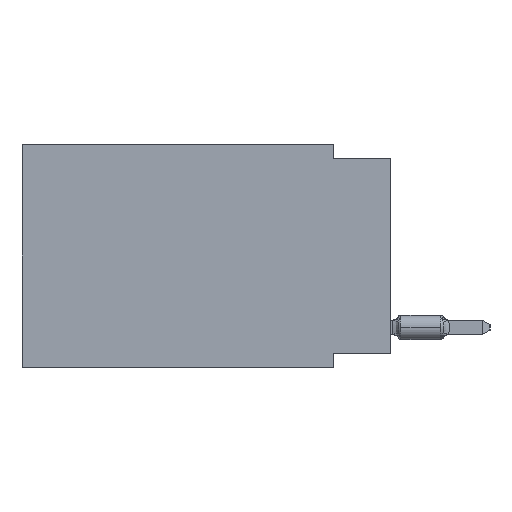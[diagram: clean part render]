
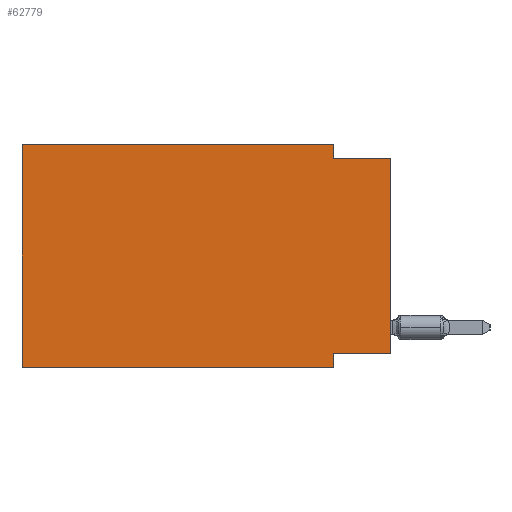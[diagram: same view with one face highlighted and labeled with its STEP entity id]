
A CAD part, left-side view. The second image highlights one B-rep face of the part: STEP entity #62779.
In plain terms, the highlighted planar face has unit normal (-1, 0, 0).
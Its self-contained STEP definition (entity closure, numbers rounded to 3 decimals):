
#2422 = LINE ( 'NONE', #65793, #82932 ) ;
#3543 = VERTEX_POINT ( 'NONE', #17332 ) ;
#3724 = VECTOR ( 'NONE', #83323, 1000. ) ;
#5546 = VECTOR ( 'NONE', #24853, 1000. ) ;
#5785 = CARTESIAN_POINT ( 'NONE',  ( 0., 2.54, -9.906 ) ) ;
#6326 = DIRECTION ( 'NONE',  ( 0., 1., 0. ) ) ;
#7982 = ORIENTED_EDGE ( 'NONE', *, *, #25823, .F. ) ;
#8582 = CARTESIAN_POINT ( 'NONE',  ( 0., 16.383, 0. ) ) ;
#11680 = CARTESIAN_POINT ( 'NONE',  ( 0., 16.383, -9.906 ) ) ;
#12291 = EDGE_CURVE ( 'NONE', #80662, #3543, #40938, .T. ) ;
#12907 = CARTESIAN_POINT ( 'NONE',  ( 0., 0., -9.271 ) ) ;
#14460 = CARTESIAN_POINT ( 'NONE',  ( 0., 2.54, 0. ) ) ;
#17332 = CARTESIAN_POINT ( 'NONE',  ( 0., 0., -0.635 ) ) ;
#18930 = AXIS2_PLACEMENT_3D ( 'NONE', #26075, #39243, #77903 ) ;
#21151 = ORIENTED_EDGE ( 'NONE', *, *, #24171, .T. ) ;
#23158 = CARTESIAN_POINT ( 'NONE',  ( 0., 2.54, -9.271 ) ) ;
#24171 = EDGE_CURVE ( 'NONE', #58174, #3543, #51066, .T. ) ;
#24853 = DIRECTION ( 'NONE',  ( 0., -1., 0. ) ) ;
#25823 = EDGE_CURVE ( 'NONE', #58174, #58140, #58614, .T. ) ;
#26075 = CARTESIAN_POINT ( 'NONE',  ( 0., 16.383, 0. ) ) ;
#26923 = CARTESIAN_POINT ( 'NONE',  ( 0., 0., -0.635 ) ) ;
#29465 = ORIENTED_EDGE ( 'NONE', *, *, #46650, .F. ) ;
#30961 = VERTEX_POINT ( 'NONE', #14460 ) ;
#31487 = DIRECTION ( 'NONE',  ( 0., 0., 1. ) ) ;
#32870 = PLANE ( 'NONE',  #18930 ) ;
#33893 = ORIENTED_EDGE ( 'NONE', *, *, #60929, .F. ) ;
#39243 = DIRECTION ( 'NONE',  ( 1., 0., 0. ) ) ;
#40882 = VERTEX_POINT ( 'NONE', #42287 ) ;
#40938 = LINE ( 'NONE', #26923, #50960 ) ;
#42287 = CARTESIAN_POINT ( 'NONE',  ( 0., 2.54, -9.906 ) ) ;
#44383 = VECTOR ( 'NONE', #31487, 1000. ) ;
#45955 = ORIENTED_EDGE ( 'NONE', *, *, #51557, .T. ) ;
#46650 = EDGE_CURVE ( 'NONE', #30961, #80662, #2422, .T. ) ;
#48649 = EDGE_CURVE ( 'NONE', #79523, #30961, #52413, .T. ) ;
#50960 = VECTOR ( 'NONE', #54100, 1000. ) ;
#51066 = LINE ( 'NONE', #77397, #3724 ) ;
#51557 = EDGE_CURVE ( 'NONE', #71599, #40882, #82225, .T. ) ;
#52413 = LINE ( 'NONE', #71969, #74443 ) ;
#52565 = VECTOR ( 'NONE', #6326, 1000. ) ;
#54100 = DIRECTION ( 'NONE',  ( 0., -1., 0. ) ) ;
#54276 = DIRECTION ( 'NONE',  ( 0., 0., -1. ) ) ;
#55542 = DIRECTION ( 'NONE',  ( 0., 0., -1. ) ) ;
#57359 = CARTESIAN_POINT ( 'NONE',  ( 0., 16.383, -9.906 ) ) ;
#58140 = VERTEX_POINT ( 'NONE', #23158 ) ;
#58174 = VERTEX_POINT ( 'NONE', #12907 ) ;
#58387 = FACE_OUTER_BOUND ( 'NONE', #65431, .T. ) ;
#58614 = LINE ( 'NONE', #76470, #52565 ) ;
#59637 = DIRECTION ( 'NONE',  ( 0., -1., 0. ) ) ;
#60111 = EDGE_CURVE ( 'NONE', #71599, #79523, #76124, .T. ) ;
#60929 = EDGE_CURVE ( 'NONE', #58140, #40882, #64034, .T. ) ;
#62779 = ADVANCED_FACE ( 'NONE', ( #58387 ), #32870, .F. ) ;
#64034 = LINE ( 'NONE', #5785, #78435 ) ;
#65431 = EDGE_LOOP ( 'NONE', ( #21151, #69616, #29465, #79855, #79095, #45955, #33893, #7982 ) ) ;
#65793 = CARTESIAN_POINT ( 'NONE',  ( 0., 2.54, 0. ) ) ;
#69616 = ORIENTED_EDGE ( 'NONE', *, *, #12291, .F. ) ;
#69751 = CARTESIAN_POINT ( 'NONE',  ( 0., 16.383, 0. ) ) ;
#71599 = VERTEX_POINT ( 'NONE', #57359 ) ;
#71969 = CARTESIAN_POINT ( 'NONE',  ( 0., 16.383, 0. ) ) ;
#74443 = VECTOR ( 'NONE', #59637, 1000. ) ;
#76124 = LINE ( 'NONE', #69751, #44383 ) ;
#76470 = CARTESIAN_POINT ( 'NONE',  ( 0., 0., -9.271 ) ) ;
#77397 = CARTESIAN_POINT ( 'NONE',  ( 0., 0., 0. ) ) ;
#77903 = DIRECTION ( 'NONE',  ( 0., 0., -1. ) ) ;
#78435 = VECTOR ( 'NONE', #55542, 1000. ) ;
#79095 = ORIENTED_EDGE ( 'NONE', *, *, #60111, .F. ) ;
#79523 = VERTEX_POINT ( 'NONE', #8582 ) ;
#79855 = ORIENTED_EDGE ( 'NONE', *, *, #48649, .F. ) ;
#80384 = CARTESIAN_POINT ( 'NONE',  ( 0., 2.54, -0.635 ) ) ;
#80662 = VERTEX_POINT ( 'NONE', #80384 ) ;
#82225 = LINE ( 'NONE', #11680, #5546 ) ;
#82932 = VECTOR ( 'NONE', #54276, 1000. ) ;
#83323 = DIRECTION ( 'NONE',  ( 0., 0., 1. ) ) ;
